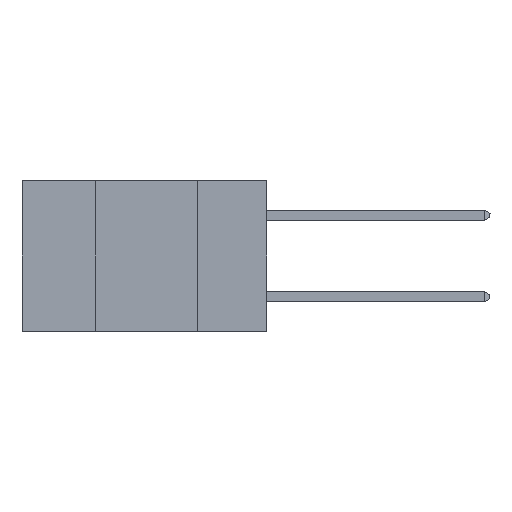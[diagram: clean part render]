
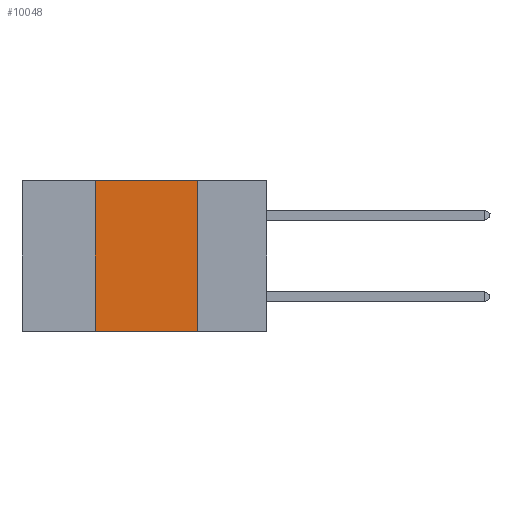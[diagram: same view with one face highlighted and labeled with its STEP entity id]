
A CAD part, left-side view. The second image highlights one B-rep face of the part: STEP entity #10048.
In plain terms, the highlighted planar face has unit normal (-1, 0, 0).
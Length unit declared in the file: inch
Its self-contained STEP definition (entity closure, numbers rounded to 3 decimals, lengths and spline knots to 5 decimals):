
#113 = DIRECTION ( 'NONE',  ( 0., 0., -1. ) ) ;
#744 = CARTESIAN_POINT ( 'NONE',  ( 0., 0.17, 0. ) ) ;
#847 = CARTESIAN_POINT ( 'NONE',  ( 0., 0.6, 0. ) ) ;
#999 = DIRECTION ( 'NONE',  ( 1., 0., 0. ) ) ;
#1981 = PLANE ( 'NONE',  #6420 ) ;
#2192 = EDGE_LOOP ( 'NONE', ( #5702, #10410, #3041, #7316 ) ) ;
#2374 = DIRECTION ( 'NONE',  ( 0., 0., 1. ) ) ;
#2444 = VECTOR ( 'NONE', #6283, 39.37008 ) ;
#2520 = DIRECTION ( 'NONE',  ( 0., 0., -1. ) ) ;
#2649 = DIRECTION ( 'NONE',  ( 0., -1., 0. ) ) ;
#2805 = CARTESIAN_POINT ( 'NONE',  ( 0., 0.6, 0. ) ) ;
#3002 = CARTESIAN_POINT ( 'NONE',  ( 0., 0.17, -0.37 ) ) ;
#3011 = LINE ( 'NONE', #10692, #2444 ) ;
#3041 = ORIENTED_EDGE ( 'NONE', *, *, #4411, .F. ) ;
#3062 = EDGE_CURVE ( 'NONE', #5731, #11080, #11201, .T. ) ;
#3209 = CARTESIAN_POINT ( 'NONE',  ( 0., 0.42, 0. ) ) ;
#3878 = VERTEX_POINT ( 'NONE', #4307 ) ;
#4307 = CARTESIAN_POINT ( 'NONE',  ( 0., 0.42, -0.37 ) ) ;
#4411 = EDGE_CURVE ( 'NONE', #3878, #5731, #6414, .T. ) ;
#4415 = FACE_OUTER_BOUND ( 'NONE', #2192, .T. ) ;
#5702 = ORIENTED_EDGE ( 'NONE', *, *, #11090, .F. ) ;
#5731 = VERTEX_POINT ( 'NONE', #3209 ) ;
#5820 = CARTESIAN_POINT ( 'NONE',  ( 0., 0.42, 0. ) ) ;
#6283 = DIRECTION ( 'NONE',  ( 0., -1., 0. ) ) ;
#6414 = LINE ( 'NONE', #5820, #7398 ) ;
#6420 = AXIS2_PLACEMENT_3D ( 'NONE', #2805, #999, #113 ) ;
#7316 = ORIENTED_EDGE ( 'NONE', *, *, #10542, .T. ) ;
#7398 = VECTOR ( 'NONE', #2374, 39.37008 ) ;
#7969 = VERTEX_POINT ( 'NONE', #3002 ) ;
#8654 = VECTOR ( 'NONE', #2520, 39.37008 ) ;
#8939 = LINE ( 'NONE', #11463, #8654 ) ;
#10048 = ADVANCED_FACE ( 'NONE', ( #4415 ), #1981, .F. ) ;
#10410 = ORIENTED_EDGE ( 'NONE', *, *, #3062, .F. ) ;
#10542 = EDGE_CURVE ( 'NONE', #3878, #7969, #3011, .T. ) ;
#10692 = CARTESIAN_POINT ( 'NONE',  ( 0., 0.6, -0.37 ) ) ;
#11080 = VERTEX_POINT ( 'NONE', #744 ) ;
#11090 = EDGE_CURVE ( 'NONE', #11080, #7969, #8939, .T. ) ;
#11201 = LINE ( 'NONE', #847, #11476 ) ;
#11463 = CARTESIAN_POINT ( 'NONE',  ( 0., 0.17, 0. ) ) ;
#11476 = VECTOR ( 'NONE', #2649, 39.37008 ) ;
